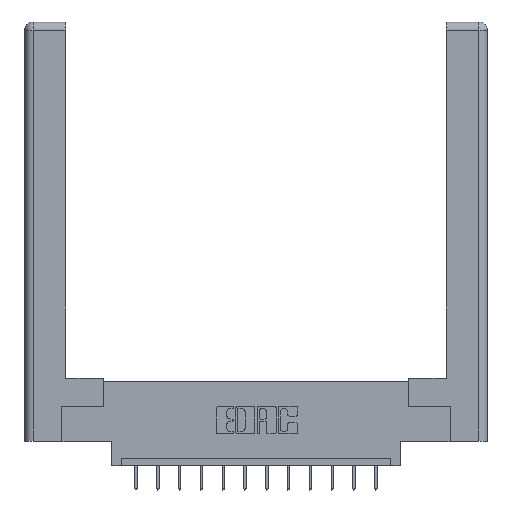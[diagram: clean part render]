
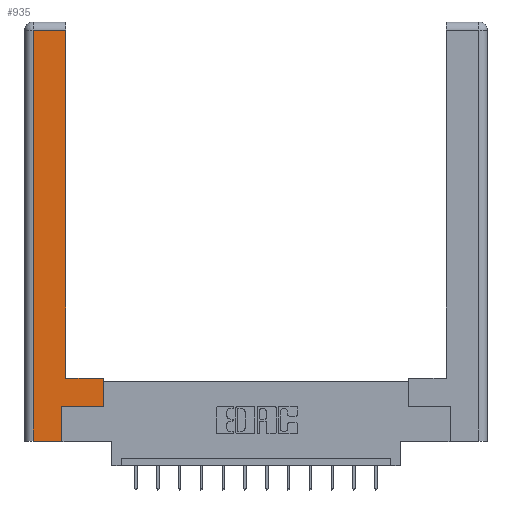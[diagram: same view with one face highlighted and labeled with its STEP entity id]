
A CAD part, top view. The second image highlights one B-rep face of the part: STEP entity #935.
In plain terms, the highlighted planar face has unit normal (0, 0, 1).
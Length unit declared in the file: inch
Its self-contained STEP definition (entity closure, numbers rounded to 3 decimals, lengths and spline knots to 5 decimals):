
#240 = EDGE_CURVE ( 'NONE', #323, #8638, #8837, .T. ) ;
#262 = EDGE_CURVE ( 'NONE', #2970, #13722, #7158, .T. ) ;
#316 = ORIENTED_EDGE ( 'NONE', *, *, #10730, .T. ) ;
#323 = VERTEX_POINT ( 'NONE', #399 ) ;
#399 = CARTESIAN_POINT ( 'NONE',  ( 0.565, 0.45, 0. ) ) ;
#403 = EDGE_CURVE ( 'NONE', #4573, #13699, #15080, .T. ) ;
#935 = ADVANCED_FACE ( 'NONE', ( #4852 ), #8721, .F. ) ;
#1073 = VECTOR ( 'NONE', #14629, 39.37008 ) ;
#1097 = CARTESIAN_POINT ( 'NONE',  ( 0.565, 0.245, 0. ) ) ;
#1475 = CARTESIAN_POINT ( 'NONE',  ( 0.295, 3., 0. ) ) ;
#1646 = CARTESIAN_POINT ( 'NONE',  ( 0.0615, 2.94, 0. ) ) ;
#1890 = DIRECTION ( 'NONE',  ( 0., 1., 0. ) ) ;
#2447 = CARTESIAN_POINT ( 'NONE',  ( 0.0615, 0., 0. ) ) ;
#2605 = DIRECTION ( 'NONE',  ( -1., 0., 0. ) ) ;
#2970 = VERTEX_POINT ( 'NONE', #7737 ) ;
#3495 = EDGE_CURVE ( 'NONE', #8638, #4573, #3651, .T. ) ;
#3641 = CARTESIAN_POINT ( 'NONE',  ( 0.565, 0.245, 0. ) ) ;
#3651 = LINE ( 'NONE', #1475, #12328 ) ;
#3992 = CARTESIAN_POINT ( 'NONE',  ( 0., 0., 0. ) ) ;
#4573 = VERTEX_POINT ( 'NONE', #12313 ) ;
#4724 = ORIENTED_EDGE ( 'NONE', *, *, #403, .T. ) ;
#4753 = ORIENTED_EDGE ( 'NONE', *, *, #14038, .T. ) ;
#4848 = DIRECTION ( 'NONE',  ( 1., 0., 0. ) ) ;
#4852 = FACE_OUTER_BOUND ( 'NONE', #9227, .T. ) ;
#5811 = CARTESIAN_POINT ( 'NONE',  ( 0.265, 0.245, 0. ) ) ;
#5871 = ORIENTED_EDGE ( 'NONE', *, *, #12196, .T. ) ;
#6519 = CARTESIAN_POINT ( 'NONE',  ( 0.265, 0.245, 0. ) ) ;
#6559 = LINE ( 'NONE', #3641, #12384 ) ;
#6809 = LINE ( 'NONE', #6519, #9603 ) ;
#6909 = EDGE_CURVE ( 'NONE', #13722, #14846, #6809, .T. ) ;
#7158 = LINE ( 'NONE', #13508, #10705 ) ;
#7250 = VECTOR ( 'NONE', #9707, 39.37008 ) ;
#7406 = VERTEX_POINT ( 'NONE', #1097 ) ;
#7717 = DIRECTION ( 'NONE',  ( 0., 1., 0. ) ) ;
#7737 = CARTESIAN_POINT ( 'NONE',  ( 0.0615, 0., 0. ) ) ;
#8638 = VERTEX_POINT ( 'NONE', #9211 ) ;
#8721 = PLANE ( 'NONE',  #11042 ) ;
#8780 = ORIENTED_EDGE ( 'NONE', *, *, #240, .T. ) ;
#8808 = CARTESIAN_POINT ( 'NONE',  ( 0.295, 0.45, 0. ) ) ;
#8837 = LINE ( 'NONE', #8808, #11104 ) ;
#9058 = CARTESIAN_POINT ( 'NONE',  ( 0.565, 0.45, 0. ) ) ;
#9211 = CARTESIAN_POINT ( 'NONE',  ( 0.295, 0.45, 0. ) ) ;
#9227 = EDGE_LOOP ( 'NONE', ( #15272, #4724, #316, #14623, #10104, #4753, #5871, #8780 ) ) ;
#9603 = VECTOR ( 'NONE', #7717, 39.37008 ) ;
#9707 = DIRECTION ( 'NONE',  ( 0., -1., 0. ) ) ;
#9997 = DIRECTION ( 'NONE',  ( 1., 0., 0. ) ) ;
#10072 = CARTESIAN_POINT ( 'NONE',  ( 0.265, 0., 0. ) ) ;
#10104 = ORIENTED_EDGE ( 'NONE', *, *, #6909, .T. ) ;
#10622 = LINE ( 'NONE', #9058, #11974 ) ;
#10705 = VECTOR ( 'NONE', #9997, 39.37008 ) ;
#10730 = EDGE_CURVE ( 'NONE', #13699, #2970, #13472, .T. ) ;
#11042 = AXIS2_PLACEMENT_3D ( 'NONE', #3992, #14790, #2605 ) ;
#11104 = VECTOR ( 'NONE', #14924, 39.37008 ) ;
#11974 = VECTOR ( 'NONE', #1890, 39.37008 ) ;
#12196 = EDGE_CURVE ( 'NONE', #7406, #323, #10622, .T. ) ;
#12313 = CARTESIAN_POINT ( 'NONE',  ( 0.295, 2.94, 0. ) ) ;
#12328 = VECTOR ( 'NONE', #13624, 39.37008 ) ;
#12384 = VECTOR ( 'NONE', #4848, 39.37008 ) ;
#13374 = CARTESIAN_POINT ( 'NONE',  ( 0.0615, 2.94, 0. ) ) ;
#13472 = LINE ( 'NONE', #2447, #7250 ) ;
#13508 = CARTESIAN_POINT ( 'NONE',  ( 0.265, 0., 0. ) ) ;
#13624 = DIRECTION ( 'NONE',  ( 0., 1., 0. ) ) ;
#13699 = VERTEX_POINT ( 'NONE', #1646 ) ;
#13722 = VERTEX_POINT ( 'NONE', #10072 ) ;
#14038 = EDGE_CURVE ( 'NONE', #14846, #7406, #6559, .T. ) ;
#14623 = ORIENTED_EDGE ( 'NONE', *, *, #262, .T. ) ;
#14629 = DIRECTION ( 'NONE',  ( -1., 0., 0. ) ) ;
#14790 = DIRECTION ( 'NONE',  ( 0., 0., -1. ) ) ;
#14846 = VERTEX_POINT ( 'NONE', #5811 ) ;
#14924 = DIRECTION ( 'NONE',  ( -1., 0., 0. ) ) ;
#15080 = LINE ( 'NONE', #13374, #1073 ) ;
#15272 = ORIENTED_EDGE ( 'NONE', *, *, #3495, .T. ) ;
